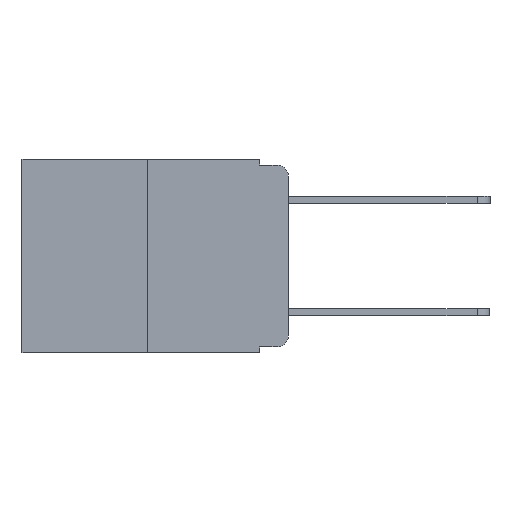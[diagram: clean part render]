
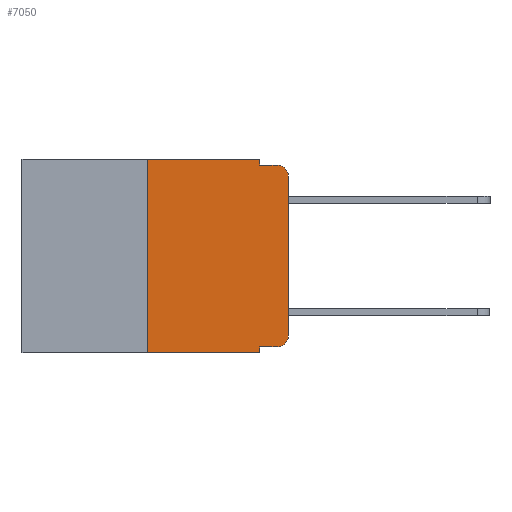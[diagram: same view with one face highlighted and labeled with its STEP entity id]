
A CAD part, left-side view. The second image highlights one B-rep face of the part: STEP entity #7050.
In plain terms, the highlighted planar face has unit normal (-1, 0, 0).
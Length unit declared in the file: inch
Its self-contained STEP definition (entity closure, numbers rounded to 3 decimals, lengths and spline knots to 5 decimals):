
#140 = CARTESIAN_POINT ( 'NONE',  ( 0., 0.25, 0. ) ) ;
#148 = CARTESIAN_POINT ( 'NONE',  ( 0., 0.473, -0.343 ) ) ;
#323 = ORIENTED_EDGE ( 'NONE', *, *, #5899, .F. ) ;
#852 = CARTESIAN_POINT ( 'NONE',  ( 0., 0., -0.313 ) ) ;
#942 = DIRECTION ( 'NONE',  ( 0., 0., -1. ) ) ;
#955 = LINE ( 'NONE', #148, #9614 ) ;
#1110 = ORIENTED_EDGE ( 'NONE', *, *, #1317, .T. ) ;
#1317 = EDGE_CURVE ( 'NONE', #7263, #7231, #955, .T. ) ;
#1325 = DIRECTION ( 'NONE',  ( 0., -1., 0. ) ) ;
#1398 = DIRECTION ( 'NONE',  ( 0., 0., -1. ) ) ;
#1633 = CARTESIAN_POINT ( 'NONE',  ( 0., 0.051, 0. ) ) ;
#2195 = VERTEX_POINT ( 'NONE', #852 ) ;
#2318 = LINE ( 'NONE', #5804, #6365 ) ;
#2663 = CARTESIAN_POINT ( 'NONE',  ( 0., 0.25, 0. ) ) ;
#2779 = CARTESIAN_POINT ( 'NONE',  ( 0., 0., -0.03 ) ) ;
#3384 = VERTEX_POINT ( 'NONE', #2779 ) ;
#3462 = LINE ( 'NONE', #6039, #7612 ) ;
#3484 = VECTOR ( 'NONE', #5381, 39.37008 ) ;
#3524 = ORIENTED_EDGE ( 'NONE', *, *, #3677, .T. ) ;
#3581 = VERTEX_POINT ( 'NONE', #5428 ) ;
#3599 = DIRECTION ( 'NONE',  ( 1., 0., 0. ) ) ;
#3677 = EDGE_CURVE ( 'NONE', #4452, #2195, #6103, .T. ) ;
#3697 = ORIENTED_EDGE ( 'NONE', *, *, #4789, .T. ) ;
#4054 = CARTESIAN_POINT ( 'NONE',  ( 0., 0.051, -0.01 ) ) ;
#4261 = PLANE ( 'NONE',  #7358 ) ;
#4264 = LINE ( 'NONE', #140, #9013 ) ;
#4382 = CARTESIAN_POINT ( 'NONE',  ( 0., 0.051, -0.01 ) ) ;
#4439 = ORIENTED_EDGE ( 'NONE', *, *, #5625, .F. ) ;
#4452 = VERTEX_POINT ( 'NONE', #8428 ) ;
#4713 = VERTEX_POINT ( 'NONE', #4382 ) ;
#4754 = VERTEX_POINT ( 'NONE', #5352 ) ;
#4789 = EDGE_CURVE ( 'NONE', #4754, #4452, #8120, .T. ) ;
#4830 = ORIENTED_EDGE ( 'NONE', *, *, #5336, .F. ) ;
#5336 = EDGE_CURVE ( 'NONE', #4754, #7231, #2318, .T. ) ;
#5352 = CARTESIAN_POINT ( 'NONE',  ( 0., 0.051, -0.333 ) ) ;
#5381 = DIRECTION ( 'NONE',  ( 0., -1., 0. ) ) ;
#5428 = CARTESIAN_POINT ( 'NONE',  ( 0., 0.051, 0. ) ) ;
#5625 = EDGE_CURVE ( 'NONE', #9680, #3581, #3462, .T. ) ;
#5804 = CARTESIAN_POINT ( 'NONE',  ( 0., 0.051, 0. ) ) ;
#5834 = AXIS2_PLACEMENT_3D ( 'NONE', #8496, #7804, #1398 ) ;
#5853 = CARTESIAN_POINT ( 'NONE',  ( 0., 0.473, 0. ) ) ;
#5899 = EDGE_CURVE ( 'NONE', #7263, #9680, #4264, .T. ) ;
#6009 = DIRECTION ( 'NONE',  ( 0., -1., 0. ) ) ;
#6013 = FACE_OUTER_BOUND ( 'NONE', #8064, .T. ) ;
#6039 = CARTESIAN_POINT ( 'NONE',  ( 0., 0.473, 0. ) ) ;
#6103 = CIRCLE ( 'NONE', #5834, 0.02 ) ;
#6365 = VECTOR ( 'NONE', #942, 39.37008 ) ;
#6372 = DIRECTION ( 'NONE',  ( 0., 0., 1. ) ) ;
#6383 = ORIENTED_EDGE ( 'NONE', *, *, #8089, .T. ) ;
#6493 = EDGE_CURVE ( 'NONE', #3581, #4713, #8541, .T. ) ;
#6710 = DIRECTION ( 'NONE',  ( 0., 0., -1. ) ) ;
#6895 = ORIENTED_EDGE ( 'NONE', *, *, #7558, .T. ) ;
#7050 = ADVANCED_FACE ( 'NONE', ( #6013 ), #4261, .F. ) ;
#7073 = EDGE_CURVE ( 'NONE', #4713, #7250, #7945, .T. ) ;
#7231 = VERTEX_POINT ( 'NONE', #8612 ) ;
#7250 = VERTEX_POINT ( 'NONE', #8489 ) ;
#7263 = VERTEX_POINT ( 'NONE', #8427 ) ;
#7292 = ORIENTED_EDGE ( 'NONE', *, *, #7073, .F. ) ;
#7358 = AXIS2_PLACEMENT_3D ( 'NONE', #5853, #3599, #7845 ) ;
#7558 = EDGE_CURVE ( 'NONE', #3384, #7250, #10909, .T. ) ;
#7612 = VECTOR ( 'NONE', #6009, 39.37008 ) ;
#7804 = DIRECTION ( 'NONE',  ( -1., 0., 0. ) ) ;
#7845 = DIRECTION ( 'NONE',  ( 0., 0., -1. ) ) ;
#7945 = LINE ( 'NONE', #4054, #9678 ) ;
#8064 = EDGE_LOOP ( 'NONE', ( #6383, #6895, #7292, #8289, #4439, #323, #1110, #4830, #3697, #3524 ) ) ;
#8089 = EDGE_CURVE ( 'NONE', #2195, #3384, #10637, .T. ) ;
#8120 = LINE ( 'NONE', #9846, #3484 ) ;
#8154 = DIRECTION ( 'NONE',  ( 0., -1., 0. ) ) ;
#8289 = ORIENTED_EDGE ( 'NONE', *, *, #6493, .F. ) ;
#8413 = DIRECTION ( 'NONE',  ( -1., 0., 0. ) ) ;
#8427 = CARTESIAN_POINT ( 'NONE',  ( 0., 0.25, -0.343 ) ) ;
#8428 = CARTESIAN_POINT ( 'NONE',  ( 0., 0.02, -0.333 ) ) ;
#8489 = CARTESIAN_POINT ( 'NONE',  ( 0., 0.02, -0.01 ) ) ;
#8492 = CARTESIAN_POINT ( 'NONE',  ( 0., 0.02, -0.03 ) ) ;
#8496 = CARTESIAN_POINT ( 'NONE',  ( 0., 0.02, -0.313 ) ) ;
#8541 = LINE ( 'NONE', #1633, #8770 ) ;
#8612 = CARTESIAN_POINT ( 'NONE',  ( 0., 0.051, -0.343 ) ) ;
#8770 = VECTOR ( 'NONE', #6710, 39.37008 ) ;
#8782 = DIRECTION ( 'NONE',  ( 0., 0., -1. ) ) ;
#9013 = VECTOR ( 'NONE', #6372, 39.37008 ) ;
#9344 = CARTESIAN_POINT ( 'NONE',  ( 0., 0., 0. ) ) ;
#9614 = VECTOR ( 'NONE', #1325, 39.37008 ) ;
#9678 = VECTOR ( 'NONE', #8154, 39.37008 ) ;
#9680 = VERTEX_POINT ( 'NONE', #2663 ) ;
#9819 = DIRECTION ( 'NONE',  ( 0., 0., 1. ) ) ;
#9846 = CARTESIAN_POINT ( 'NONE',  ( 0., 0.051, -0.333 ) ) ;
#10183 = VECTOR ( 'NONE', #9819, 39.37008 ) ;
#10488 = AXIS2_PLACEMENT_3D ( 'NONE', #8492, #8413, #8782 ) ;
#10637 = LINE ( 'NONE', #9344, #10183 ) ;
#10909 = CIRCLE ( 'NONE', #10488, 0.02 ) ;
